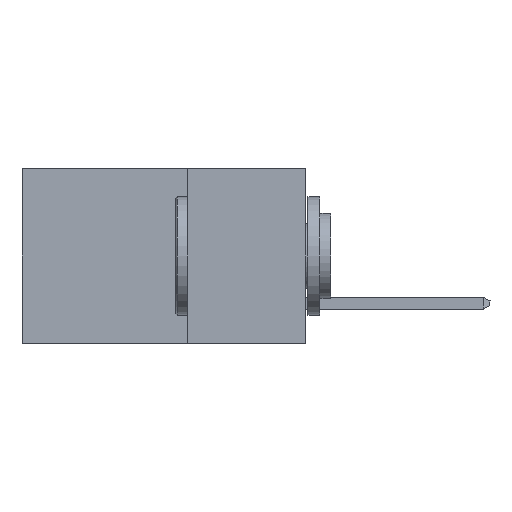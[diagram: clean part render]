
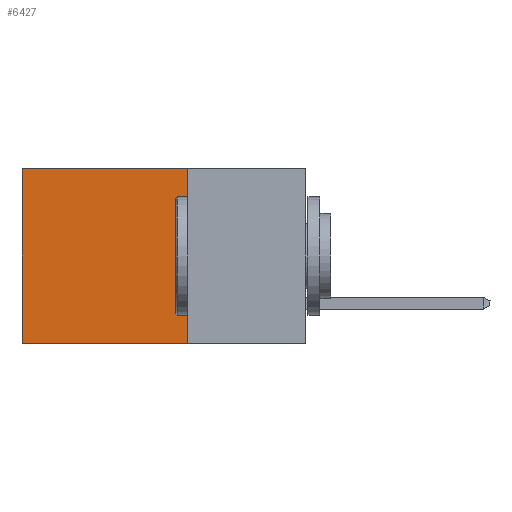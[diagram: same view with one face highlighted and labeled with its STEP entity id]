
A CAD part, left-side view. The second image highlights one B-rep face of the part: STEP entity #6427.
In plain terms, the highlighted planar face has unit normal (-1, 0, 0).
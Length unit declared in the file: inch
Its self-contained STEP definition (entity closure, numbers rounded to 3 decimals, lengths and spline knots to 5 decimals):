
#102 = ORIENTED_EDGE ( 'NONE', *, *, #5392, .F. ) ;
#1664 = LINE ( 'NONE', #12600, #17007 ) ;
#2857 = VECTOR ( 'NONE', #13133, 39.37008 ) ;
#3212 = VERTEX_POINT ( 'NONE', #8968 ) ;
#4009 = ORIENTED_EDGE ( 'NONE', *, *, #8324, .T. ) ;
#4896 = CARTESIAN_POINT ( 'NONE',  ( 0.298, 0.25, 0. ) ) ;
#4963 = VERTEX_POINT ( 'NONE', #8148 ) ;
#5149 = AXIS2_PLACEMENT_3D ( 'NONE', #4896, #16697, #16758 ) ;
#5184 = CARTESIAN_POINT ( 'NONE',  ( 0.298, 0.25, 0. ) ) ;
#5392 = EDGE_CURVE ( 'NONE', #4963, #3212, #9688, .T. ) ;
#6126 = LINE ( 'NONE', #14822, #13750 ) ;
#6427 = ADVANCED_FACE ( 'NONE', ( #10328 ), #15369, .F. ) ;
#6611 = EDGE_LOOP ( 'NONE', ( #16610, #102, #16038, #4009 ) ) ;
#7933 = EDGE_CURVE ( 'NONE', #9961, #4963, #6126, .T. ) ;
#8148 = CARTESIAN_POINT ( 'NONE',  ( 0.298, 0.25, -0.37 ) ) ;
#8324 = EDGE_CURVE ( 'NONE', #9961, #16430, #15421, .T. ) ;
#8524 = DIRECTION ( 'NONE',  ( 0., 0., -1. ) ) ;
#8968 = CARTESIAN_POINT ( 'NONE',  ( 0.298, 0.6, -0.37 ) ) ;
#9215 = VECTOR ( 'NONE', #16576, 39.37008 ) ;
#9688 = LINE ( 'NONE', #11823, #2857 ) ;
#9961 = VERTEX_POINT ( 'NONE', #13348 ) ;
#10328 = FACE_OUTER_BOUND ( 'NONE', #6611, .T. ) ;
#11394 = DIRECTION ( 'NONE',  ( 0., 0., -1. ) ) ;
#11823 = CARTESIAN_POINT ( 'NONE',  ( 0.298, 0.25, -0.37 ) ) ;
#12600 = CARTESIAN_POINT ( 'NONE',  ( 0.298, 0.6, 0. ) ) ;
#13133 = DIRECTION ( 'NONE',  ( 0., 1., 0. ) ) ;
#13348 = CARTESIAN_POINT ( 'NONE',  ( 0.298, 0.25, 0. ) ) ;
#13750 = VECTOR ( 'NONE', #8524, 39.37008 ) ;
#14822 = CARTESIAN_POINT ( 'NONE',  ( 0.298, 0.25, 0. ) ) ;
#15369 = PLANE ( 'NONE',  #5149 ) ;
#15421 = LINE ( 'NONE', #5184, #9215 ) ;
#16038 = ORIENTED_EDGE ( 'NONE', *, *, #7933, .F. ) ;
#16218 = EDGE_CURVE ( 'NONE', #16430, #3212, #1664, .T. ) ;
#16430 = VERTEX_POINT ( 'NONE', #16872 ) ;
#16576 = DIRECTION ( 'NONE',  ( 0., 1., 0. ) ) ;
#16610 = ORIENTED_EDGE ( 'NONE', *, *, #16218, .T. ) ;
#16697 = DIRECTION ( 'NONE',  ( 1., 0., 0. ) ) ;
#16758 = DIRECTION ( 'NONE',  ( 0., 0., -1. ) ) ;
#16872 = CARTESIAN_POINT ( 'NONE',  ( 0.298, 0.6, 0. ) ) ;
#17007 = VECTOR ( 'NONE', #11394, 39.37008 ) ;
